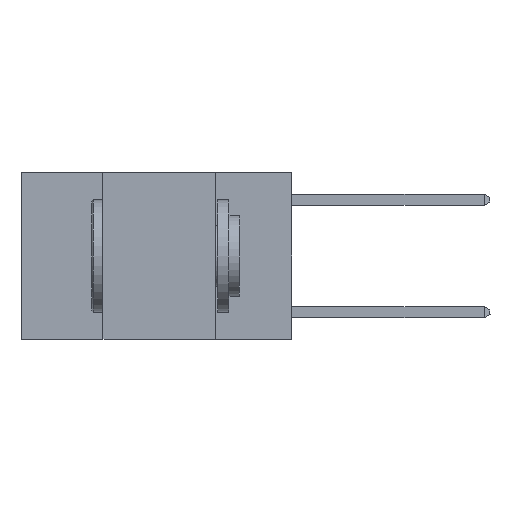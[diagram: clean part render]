
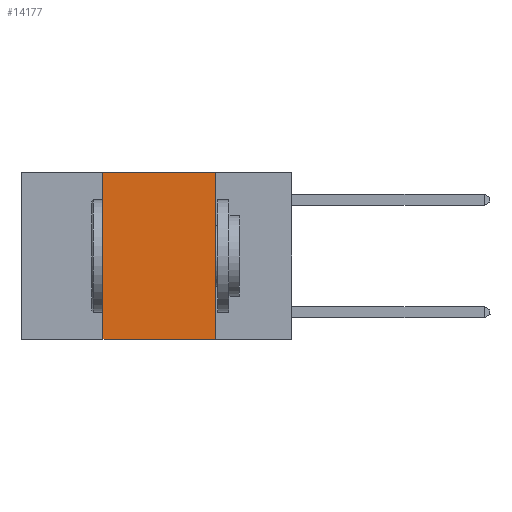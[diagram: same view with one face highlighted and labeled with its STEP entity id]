
A CAD part, left-side view. The second image highlights one B-rep face of the part: STEP entity #14177.
In plain terms, the highlighted planar face has unit normal (-1, 0, 0).
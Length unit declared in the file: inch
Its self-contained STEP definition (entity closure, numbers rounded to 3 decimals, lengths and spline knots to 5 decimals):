
#301 = ORIENTED_EDGE ( 'NONE', *, *, #7698, .F. ) ;
#339 = FACE_OUTER_BOUND ( 'NONE', #8118, .T. ) ;
#1610 = CARTESIAN_POINT ( 'NONE',  ( 0., 0.6, 0. ) ) ;
#1829 = VECTOR ( 'NONE', #5632, 39.37008 ) ;
#1899 = EDGE_CURVE ( 'NONE', #10867, #3232, #10482, .T. ) ;
#1967 = ORIENTED_EDGE ( 'NONE', *, *, #2506, .F. ) ;
#2230 = VECTOR ( 'NONE', #6479, 39.37008 ) ;
#2506 = EDGE_CURVE ( 'NONE', #10867, #16625, #10812, .T. ) ;
#2707 = CARTESIAN_POINT ( 'NONE',  ( 0., 0.42, 0. ) ) ;
#3043 = DIRECTION ( 'NONE',  ( 1., 0., 0. ) ) ;
#3232 = VERTEX_POINT ( 'NONE', #4418 ) ;
#3887 = LINE ( 'NONE', #1610, #1829 ) ;
#3928 = DIRECTION ( 'NONE',  ( 0., 0., 1. ) ) ;
#4418 = CARTESIAN_POINT ( 'NONE',  ( 0., 0.17, -0.37 ) ) ;
#4670 = VECTOR ( 'NONE', #11131, 39.37008 ) ;
#4910 = VECTOR ( 'NONE', #3928, 39.37008 ) ;
#5632 = DIRECTION ( 'NONE',  ( 0., -1., 0. ) ) ;
#6218 = ORIENTED_EDGE ( 'NONE', *, *, #15555, .F. ) ;
#6479 = DIRECTION ( 'NONE',  ( 0., -1., 0. ) ) ;
#6871 = DIRECTION ( 'NONE',  ( 0., 0., -1. ) ) ;
#7121 = CARTESIAN_POINT ( 'NONE',  ( 0., 0.17, 0. ) ) ;
#7429 = CARTESIAN_POINT ( 'NONE',  ( 0., 0.6, -0.37 ) ) ;
#7511 = CARTESIAN_POINT ( 'NONE',  ( 0., 0.42, 0. ) ) ;
#7698 = EDGE_CURVE ( 'NONE', #16625, #9220, #3887, .T. ) ;
#8026 = AXIS2_PLACEMENT_3D ( 'NONE', #8342, #3043, #6871 ) ;
#8118 = EDGE_LOOP ( 'NONE', ( #6218, #301, #1967, #10771 ) ) ;
#8342 = CARTESIAN_POINT ( 'NONE',  ( 0., 0.6, 0. ) ) ;
#9220 = VERTEX_POINT ( 'NONE', #12785 ) ;
#9392 = PLANE ( 'NONE',  #8026 ) ;
#10482 = LINE ( 'NONE', #7429, #2230 ) ;
#10771 = ORIENTED_EDGE ( 'NONE', *, *, #1899, .T. ) ;
#10812 = LINE ( 'NONE', #2707, #4910 ) ;
#10867 = VERTEX_POINT ( 'NONE', #13758 ) ;
#11131 = DIRECTION ( 'NONE',  ( 0., 0., -1. ) ) ;
#12182 = LINE ( 'NONE', #7121, #4670 ) ;
#12785 = CARTESIAN_POINT ( 'NONE',  ( 0., 0.17, 0. ) ) ;
#13758 = CARTESIAN_POINT ( 'NONE',  ( 0., 0.42, -0.37 ) ) ;
#14177 = ADVANCED_FACE ( 'NONE', ( #339 ), #9392, .F. ) ;
#15555 = EDGE_CURVE ( 'NONE', #9220, #3232, #12182, .T. ) ;
#16625 = VERTEX_POINT ( 'NONE', #7511 ) ;
